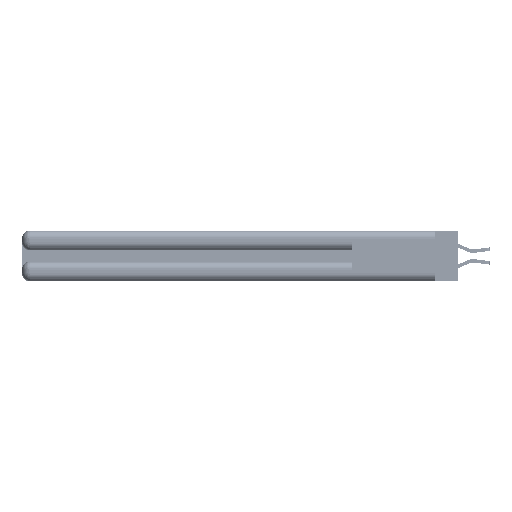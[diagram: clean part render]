
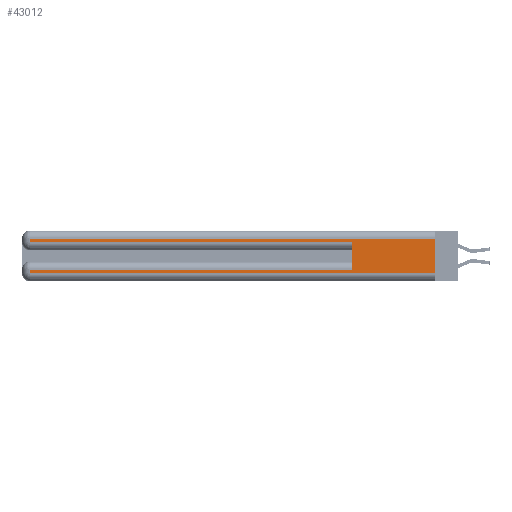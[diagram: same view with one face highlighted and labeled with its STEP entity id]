
A CAD part, left-side view. The second image highlights one B-rep face of the part: STEP entity #43012.
In plain terms, the highlighted planar face has unit normal (-1, 0, 0).
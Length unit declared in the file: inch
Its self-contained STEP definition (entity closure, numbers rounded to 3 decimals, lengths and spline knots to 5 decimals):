
#858 = ORIENTED_EDGE ( 'NONE', *, *, #23965, .F. ) ;
#1182 = CARTESIAN_POINT ( 'NONE',  ( 0., 2.94, 0.06 ) ) ;
#3644 = DIRECTION ( 'NONE',  ( 0., 0., -1. ) ) ;
#5436 = CARTESIAN_POINT ( 'NONE',  ( 0., 2.94, 0.31 ) ) ;
#5663 = VERTEX_POINT ( 'NONE', #51716 ) ;
#6224 = DIRECTION ( 'NONE',  ( 0., 0., -1. ) ) ;
#6313 = VECTOR ( 'NONE', #3644, 39.37008 ) ;
#6588 = CARTESIAN_POINT ( 'NONE',  ( 0., 2.94, 0.37 ) ) ;
#7214 = VECTOR ( 'NONE', #10283, 39.37008 ) ;
#7306 = CARTESIAN_POINT ( 'NONE',  ( 0., 0., 0.06 ) ) ;
#8889 = ORIENTED_EDGE ( 'NONE', *, *, #9468, .F. ) ;
#9310 = CARTESIAN_POINT ( 'NONE',  ( 0., 0., 0.285 ) ) ;
#9326 = VECTOR ( 'NONE', #28727, 39.37008 ) ;
#9468 = EDGE_CURVE ( 'NONE', #18930, #5663, #44401, .T. ) ;
#9689 = EDGE_LOOP ( 'NONE', ( #858, #55378, #55971, #36458, #8889, #51911, #44549, #55856 ) ) ;
#10283 = DIRECTION ( 'NONE',  ( 0., 0., -1. ) ) ;
#10290 = PLANE ( 'NONE',  #35685 ) ;
#10358 = VERTEX_POINT ( 'NONE', #5436 ) ;
#11706 = DIRECTION ( 'NONE',  ( 0., 0., 1. ) ) ;
#13000 = VERTEX_POINT ( 'NONE', #21609 ) ;
#14696 = CARTESIAN_POINT ( 'NONE',  ( 0., 0., 0.31 ) ) ;
#15290 = VERTEX_POINT ( 'NONE', #25571 ) ;
#15996 = LINE ( 'NONE', #36105, #7214 ) ;
#16567 = CARTESIAN_POINT ( 'NONE',  ( 0., 2.94, 0.285 ) ) ;
#16673 = CARTESIAN_POINT ( 'NONE',  ( 0., 0.6, 0.085 ) ) ;
#18524 = EDGE_CURVE ( 'NONE', #15290, #40956, #44991, .T. ) ;
#18930 = VERTEX_POINT ( 'NONE', #16673 ) ;
#21545 = VERTEX_POINT ( 'NONE', #25015 ) ;
#21609 = CARTESIAN_POINT ( 'NONE',  ( 0., 0., 0.06 ) ) ;
#22567 = DIRECTION ( 'NONE',  ( 0., -1., 0. ) ) ;
#23361 = EDGE_CURVE ( 'NONE', #21545, #10358, #24243, .T. ) ;
#23764 = DIRECTION ( 'NONE',  ( 1., 0., 0. ) ) ;
#23965 = EDGE_CURVE ( 'NONE', #21545, #13000, #15996, .T. ) ;
#24243 = LINE ( 'NONE', #14696, #48645 ) ;
#25015 = CARTESIAN_POINT ( 'NONE',  ( 0., 0., 0.31 ) ) ;
#25018 = CARTESIAN_POINT ( 'NONE',  ( 0., 0.6, 0.145 ) ) ;
#25571 = CARTESIAN_POINT ( 'NONE',  ( 0., 2.94, 0.085 ) ) ;
#25831 = VECTOR ( 'NONE', #22567, 39.37008 ) ;
#25913 = DIRECTION ( 'NONE',  ( 0., 1., 0. ) ) ;
#28309 = DIRECTION ( 'NONE',  ( 0., 0., -1. ) ) ;
#28727 = DIRECTION ( 'NONE',  ( 0., -1., 0. ) ) ;
#29710 = VECTOR ( 'NONE', #25913, 39.37008 ) ;
#29885 = CARTESIAN_POINT ( 'NONE',  ( 0., 0., 0.085 ) ) ;
#31526 = VECTOR ( 'NONE', #11706, 39.37008 ) ;
#32739 = EDGE_CURVE ( 'NONE', #18930, #15290, #48734, .T. ) ;
#35153 = LINE ( 'NONE', #7306, #9326 ) ;
#35685 = AXIS2_PLACEMENT_3D ( 'NONE', #41223, #23764, #28309 ) ;
#36105 = CARTESIAN_POINT ( 'NONE',  ( 0., 0., 0.37 ) ) ;
#36458 = ORIENTED_EDGE ( 'NONE', *, *, #37743, .T. ) ;
#37743 = EDGE_CURVE ( 'NONE', #45913, #5663, #38096, .T. ) ;
#38096 = LINE ( 'NONE', #9310, #25831 ) ;
#39082 = LINE ( 'NONE', #6588, #56032 ) ;
#40477 = EDGE_CURVE ( 'NONE', #40956, #13000, #35153, .T. ) ;
#40956 = VERTEX_POINT ( 'NONE', #1182 ) ;
#41223 = CARTESIAN_POINT ( 'NONE',  ( 0., 0., 0.37 ) ) ;
#43012 = ADVANCED_FACE ( 'NONE', ( #43738 ), #10290, .F. ) ;
#43738 = FACE_OUTER_BOUND ( 'NONE', #9689, .T. ) ;
#44401 = LINE ( 'NONE', #25018, #31526 ) ;
#44549 = ORIENTED_EDGE ( 'NONE', *, *, #18524, .T. ) ;
#44991 = LINE ( 'NONE', #55598, #6313 ) ;
#45443 = DIRECTION ( 'NONE',  ( 0., 1., 0. ) ) ;
#45527 = EDGE_CURVE ( 'NONE', #10358, #45913, #39082, .T. ) ;
#45913 = VERTEX_POINT ( 'NONE', #16567 ) ;
#48645 = VECTOR ( 'NONE', #45443, 39.37008 ) ;
#48734 = LINE ( 'NONE', #29885, #29710 ) ;
#51716 = CARTESIAN_POINT ( 'NONE',  ( 0., 0.6, 0.285 ) ) ;
#51911 = ORIENTED_EDGE ( 'NONE', *, *, #32739, .T. ) ;
#55378 = ORIENTED_EDGE ( 'NONE', *, *, #23361, .T. ) ;
#55598 = CARTESIAN_POINT ( 'NONE',  ( 0., 2.94, 0.37 ) ) ;
#55856 = ORIENTED_EDGE ( 'NONE', *, *, #40477, .T. ) ;
#55971 = ORIENTED_EDGE ( 'NONE', *, *, #45527, .T. ) ;
#56032 = VECTOR ( 'NONE', #6224, 39.37008 ) ;
